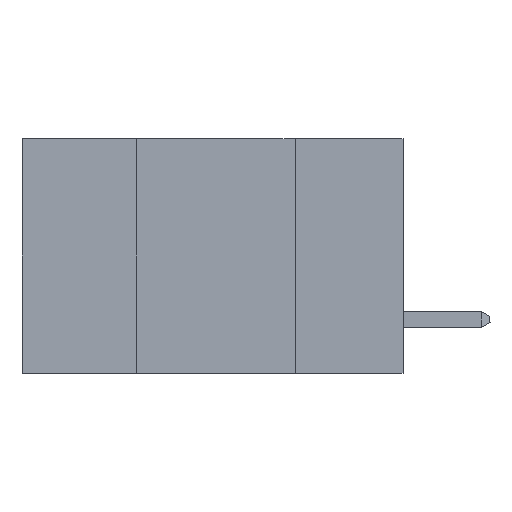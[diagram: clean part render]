
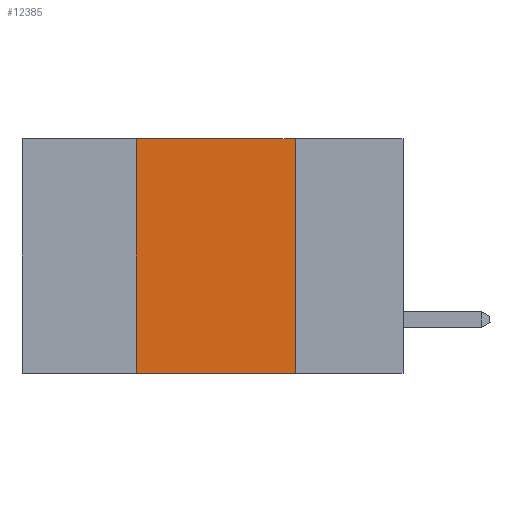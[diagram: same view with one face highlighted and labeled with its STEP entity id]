
A CAD part, left-side view. The second image highlights one B-rep face of the part: STEP entity #12385.
In plain terms, the highlighted planar face has unit normal (-1, 0, 0).
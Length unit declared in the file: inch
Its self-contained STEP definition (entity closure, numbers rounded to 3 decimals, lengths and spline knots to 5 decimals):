
#366 = VERTEX_POINT ( 'NONE', #4408 ) ;
#630 = ORIENTED_EDGE ( 'NONE', *, *, #8138, .F. ) ;
#995 = ORIENTED_EDGE ( 'NONE', *, *, #9394, .T. ) ;
#1758 = ORIENTED_EDGE ( 'NONE', *, *, #7495, .F. ) ;
#1862 = DIRECTION ( 'NONE',  ( 0., -1., 0. ) ) ;
#3795 = CARTESIAN_POINT ( 'NONE',  ( 0., 0.17, -0.37 ) ) ;
#4408 = CARTESIAN_POINT ( 'NONE',  ( 0., 0.17, 0. ) ) ;
#4888 = LINE ( 'NONE', #17791, #11425 ) ;
#5346 = DIRECTION ( 'NONE',  ( 0., 0., -1. ) ) ;
#5903 = CARTESIAN_POINT ( 'NONE',  ( 0., 0.42, 0. ) ) ;
#6589 = CARTESIAN_POINT ( 'NONE',  ( 0., 0.42, -0.37 ) ) ;
#6713 = VECTOR ( 'NONE', #5346, 39.37008 ) ;
#7495 = EDGE_CURVE ( 'NONE', #7906, #14610, #9912, .T. ) ;
#7906 = VERTEX_POINT ( 'NONE', #6589 ) ;
#8138 = EDGE_CURVE ( 'NONE', #366, #13802, #13021, .T. ) ;
#9173 = VECTOR ( 'NONE', #12171, 39.37008 ) ;
#9394 = EDGE_CURVE ( 'NONE', #7906, #13802, #4888, .T. ) ;
#9601 = EDGE_LOOP ( 'NONE', ( #630, #15895, #1758, #995 ) ) ;
#9912 = LINE ( 'NONE', #5903, #9173 ) ;
#10807 = FACE_OUTER_BOUND ( 'NONE', #9601, .T. ) ;
#10911 = LINE ( 'NONE', #18753, #16694 ) ;
#11425 = VECTOR ( 'NONE', #17860, 39.37008 ) ;
#11623 = CARTESIAN_POINT ( 'NONE',  ( 0., 0.17, 0. ) ) ;
#12171 = DIRECTION ( 'NONE',  ( 0., 0., 1. ) ) ;
#12385 = ADVANCED_FACE ( 'NONE', ( #10807 ), #13338, .F. ) ;
#13021 = LINE ( 'NONE', #11623, #6713 ) ;
#13338 = PLANE ( 'NONE',  #13797 ) ;
#13797 = AXIS2_PLACEMENT_3D ( 'NONE', #17855, #16380, #18311 ) ;
#13802 = VERTEX_POINT ( 'NONE', #3795 ) ;
#14610 = VERTEX_POINT ( 'NONE', #17919 ) ;
#15895 = ORIENTED_EDGE ( 'NONE', *, *, #17901, .F. ) ;
#16380 = DIRECTION ( 'NONE',  ( 1., 0., 0. ) ) ;
#16694 = VECTOR ( 'NONE', #1862, 39.37008 ) ;
#17791 = CARTESIAN_POINT ( 'NONE',  ( 0., 0.6, -0.37 ) ) ;
#17855 = CARTESIAN_POINT ( 'NONE',  ( 0., 0.6, 0. ) ) ;
#17860 = DIRECTION ( 'NONE',  ( 0., -1., 0. ) ) ;
#17901 = EDGE_CURVE ( 'NONE', #14610, #366, #10911, .T. ) ;
#17919 = CARTESIAN_POINT ( 'NONE',  ( 0., 0.42, 0. ) ) ;
#18311 = DIRECTION ( 'NONE',  ( 0., 0., -1. ) ) ;
#18753 = CARTESIAN_POINT ( 'NONE',  ( 0., 0.6, 0. ) ) ;
